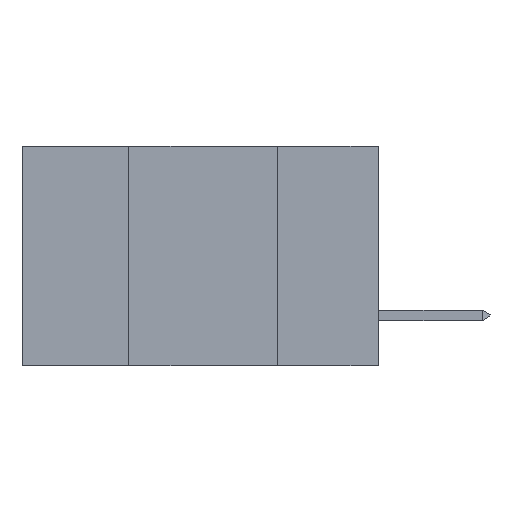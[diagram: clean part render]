
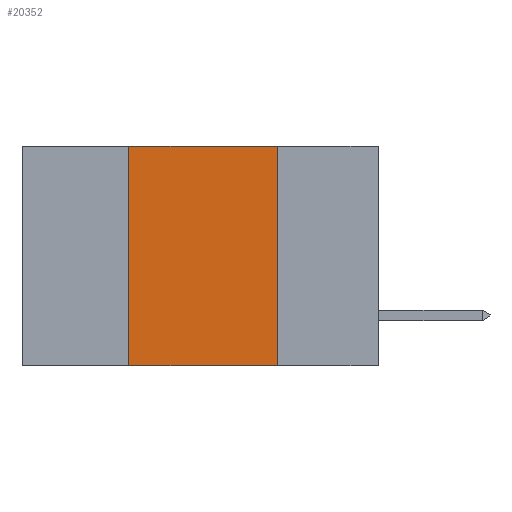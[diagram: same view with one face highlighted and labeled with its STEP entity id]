
A CAD part, left-side view. The second image highlights one B-rep face of the part: STEP entity #20352.
In plain terms, the highlighted planar face has unit normal (-1, 0, 0).
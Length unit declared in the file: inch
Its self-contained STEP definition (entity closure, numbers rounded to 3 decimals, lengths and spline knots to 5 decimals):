
#550 = VERTEX_POINT ( 'NONE', #10604 ) ;
#597 = ORIENTED_EDGE ( 'NONE', *, *, #4513, .F. ) ;
#1532 = PLANE ( 'NONE',  #4378 ) ;
#2164 = CARTESIAN_POINT ( 'NONE',  ( 0., 0.17, 0. ) ) ;
#3894 = FACE_OUTER_BOUND ( 'NONE', #4155, .T. ) ;
#4155 = EDGE_LOOP ( 'NONE', ( #21238, #597, #10430, #15194 ) ) ;
#4378 = AXIS2_PLACEMENT_3D ( 'NONE', #28482, #8979, #8754 ) ;
#4513 = EDGE_CURVE ( 'NONE', #26987, #550, #14066, .T. ) ;
#4850 = VECTOR ( 'NONE', #10970, 39.37008 ) ;
#6371 = EDGE_CURVE ( 'NONE', #550, #7896, #25721, .T. ) ;
#7598 = VECTOR ( 'NONE', #19368, 39.37008 ) ;
#7896 = VERTEX_POINT ( 'NONE', #23455 ) ;
#8754 = DIRECTION ( 'NONE',  ( 0., 0., -1. ) ) ;
#8979 = DIRECTION ( 'NONE',  ( 1., 0., 0. ) ) ;
#10430 = ORIENTED_EDGE ( 'NONE', *, *, #18997, .F. ) ;
#10604 = CARTESIAN_POINT ( 'NONE',  ( 0., 0.17, 0. ) ) ;
#10746 = CARTESIAN_POINT ( 'NONE',  ( 0., 0.42, -0.37 ) ) ;
#10970 = DIRECTION ( 'NONE',  ( 0., 0., 1. ) ) ;
#12621 = CARTESIAN_POINT ( 'NONE',  ( 0., 0.6, -0.37 ) ) ;
#12789 = CARTESIAN_POINT ( 'NONE',  ( 0., 0.42, 0. ) ) ;
#13734 = VERTEX_POINT ( 'NONE', #10746 ) ;
#14066 = LINE ( 'NONE', #29163, #7598 ) ;
#15194 = ORIENTED_EDGE ( 'NONE', *, *, #19609, .T. ) ;
#15712 = VECTOR ( 'NONE', #30073, 39.37008 ) ;
#18997 = EDGE_CURVE ( 'NONE', #13734, #26987, #24239, .T. ) ;
#19368 = DIRECTION ( 'NONE',  ( 0., -1., 0. ) ) ;
#19609 = EDGE_CURVE ( 'NONE', #13734, #7896, #22953, .T. ) ;
#20352 = ADVANCED_FACE ( 'NONE', ( #3894 ), #1532, .F. ) ;
#21238 = ORIENTED_EDGE ( 'NONE', *, *, #6371, .F. ) ;
#22953 = LINE ( 'NONE', #12621, #15712 ) ;
#23299 = CARTESIAN_POINT ( 'NONE',  ( 0., 0.42, 0. ) ) ;
#23455 = CARTESIAN_POINT ( 'NONE',  ( 0., 0.17, -0.37 ) ) ;
#24031 = DIRECTION ( 'NONE',  ( 0., 0., -1. ) ) ;
#24201 = VECTOR ( 'NONE', #24031, 39.37008 ) ;
#24239 = LINE ( 'NONE', #23299, #4850 ) ;
#25721 = LINE ( 'NONE', #2164, #24201 ) ;
#26987 = VERTEX_POINT ( 'NONE', #12789 ) ;
#28482 = CARTESIAN_POINT ( 'NONE',  ( 0., 0.6, 0. ) ) ;
#29163 = CARTESIAN_POINT ( 'NONE',  ( 0., 0.6, 0. ) ) ;
#30073 = DIRECTION ( 'NONE',  ( 0., -1., 0. ) ) ;
